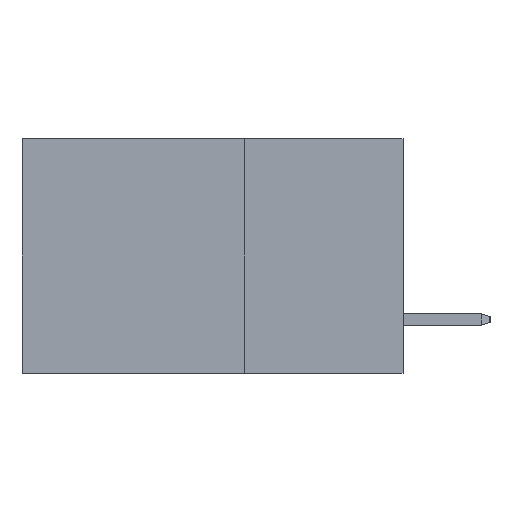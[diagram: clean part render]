
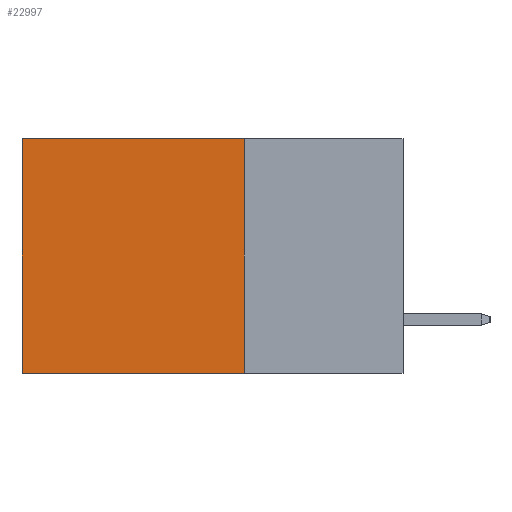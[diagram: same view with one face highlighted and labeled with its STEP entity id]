
A CAD part, left-side view. The second image highlights one B-rep face of the part: STEP entity #22997.
In plain terms, the highlighted planar face has unit normal (-1, 0, 0).
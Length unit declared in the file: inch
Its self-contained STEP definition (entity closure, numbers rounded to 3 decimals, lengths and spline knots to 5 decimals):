
#431 = CARTESIAN_POINT ( 'NONE',  ( 0.2875, 0.6, -0.37 ) ) ;
#1972 = LINE ( 'NONE', #12484, #22641 ) ;
#2899 = LINE ( 'NONE', #10946, #3637 ) ;
#3621 = ORIENTED_EDGE ( 'NONE', *, *, #5208, .F. ) ;
#3637 = VECTOR ( 'NONE', #25047, 39.37008 ) ;
#3745 = PLANE ( 'NONE',  #21297 ) ;
#3869 = DIRECTION ( 'NONE',  ( 1., 0., 0. ) ) ;
#3888 = CARTESIAN_POINT ( 'NONE',  ( 0.2875, 0.6, 0. ) ) ;
#5208 = EDGE_CURVE ( 'NONE', #11166, #19790, #2899, .T. ) ;
#5266 = VERTEX_POINT ( 'NONE', #7495 ) ;
#5604 = CARTESIAN_POINT ( 'NONE',  ( 0.2875, 0.6, 0. ) ) ;
#5681 = VERTEX_POINT ( 'NONE', #5604 ) ;
#5818 = EDGE_CURVE ( 'NONE', #5681, #19790, #24066, .T. ) ;
#5970 = FACE_OUTER_BOUND ( 'NONE', #11823, .T. ) ;
#7495 = CARTESIAN_POINT ( 'NONE',  ( 0.2875, 0.25, 0. ) ) ;
#8318 = ORIENTED_EDGE ( 'NONE', *, *, #5818, .T. ) ;
#9809 = DIRECTION ( 'NONE',  ( 0., 0., -1. ) ) ;
#10946 = CARTESIAN_POINT ( 'NONE',  ( 0.2875, 0.25, -0.37 ) ) ;
#11166 = VERTEX_POINT ( 'NONE', #21625 ) ;
#11823 = EDGE_LOOP ( 'NONE', ( #8318, #3621, #19216, #18984 ) ) ;
#12484 = CARTESIAN_POINT ( 'NONE',  ( 0.2875, 0.25, 0. ) ) ;
#12515 = DIRECTION ( 'NONE',  ( 0., 1., 0. ) ) ;
#12600 = EDGE_CURVE ( 'NONE', #5266, #5681, #1972, .T. ) ;
#13897 = CARTESIAN_POINT ( 'NONE',  ( 0.2875, 0.25, 0. ) ) ;
#14633 = VECTOR ( 'NONE', #17872, 39.37008 ) ;
#17734 = CARTESIAN_POINT ( 'NONE',  ( 0.2875, 0.25, 0. ) ) ;
#17872 = DIRECTION ( 'NONE',  ( 0., 0., -1. ) ) ;
#18369 = VECTOR ( 'NONE', #9809, 39.37008 ) ;
#18984 = ORIENTED_EDGE ( 'NONE', *, *, #12600, .T. ) ;
#19216 = ORIENTED_EDGE ( 'NONE', *, *, #24028, .F. ) ;
#19790 = VERTEX_POINT ( 'NONE', #431 ) ;
#19830 = DIRECTION ( 'NONE',  ( 0., 0., -1. ) ) ;
#21297 = AXIS2_PLACEMENT_3D ( 'NONE', #13897, #3869, #19830 ) ;
#21625 = CARTESIAN_POINT ( 'NONE',  ( 0.2875, 0.25, -0.37 ) ) ;
#22641 = VECTOR ( 'NONE', #12515, 39.37008 ) ;
#22997 = ADVANCED_FACE ( 'NONE', ( #5970 ), #3745, .F. ) ;
#24028 = EDGE_CURVE ( 'NONE', #5266, #11166, #25656, .T. ) ;
#24066 = LINE ( 'NONE', #3888, #14633 ) ;
#25047 = DIRECTION ( 'NONE',  ( 0., 1., 0. ) ) ;
#25656 = LINE ( 'NONE', #17734, #18369 ) ;
